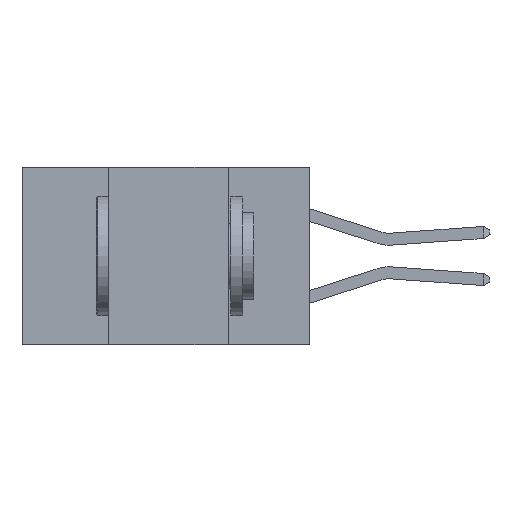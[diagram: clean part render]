
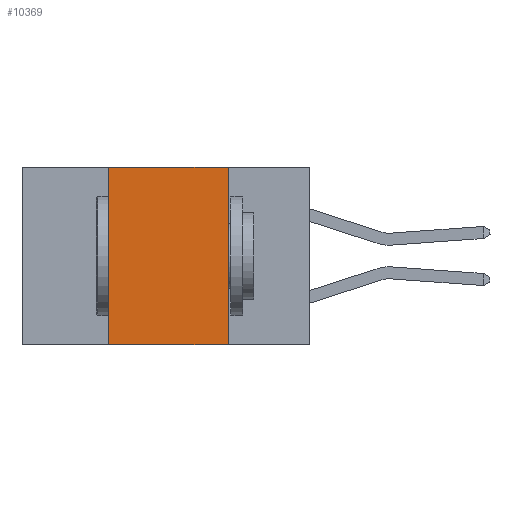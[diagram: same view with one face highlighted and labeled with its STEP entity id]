
A CAD part, left-side view. The second image highlights one B-rep face of the part: STEP entity #10369.
In plain terms, the highlighted planar face has unit normal (-1, 0, 0).
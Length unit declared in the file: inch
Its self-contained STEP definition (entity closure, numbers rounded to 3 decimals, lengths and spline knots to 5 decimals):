
#608 = DIRECTION ( 'NONE',  ( 0., -1., 0. ) ) ;
#1978 = VECTOR ( 'NONE', #22220, 39.37008 ) ;
#2486 = EDGE_CURVE ( 'NONE', #22380, #10706, #23877, .T. ) ;
#3511 = CARTESIAN_POINT ( 'NONE',  ( 0., 0.17, -0.37 ) ) ;
#4095 = CARTESIAN_POINT ( 'NONE',  ( 0., 0.42, -0.37 ) ) ;
#6187 = ORIENTED_EDGE ( 'NONE', *, *, #8507, .T. ) ;
#6933 = AXIS2_PLACEMENT_3D ( 'NONE', #25774, #12176, #10181 ) ;
#7000 = CARTESIAN_POINT ( 'NONE',  ( 0., 0.17, 0. ) ) ;
#7050 = ORIENTED_EDGE ( 'NONE', *, *, #11353, .F. ) ;
#7614 = DIRECTION ( 'NONE',  ( 0., 0., -1. ) ) ;
#8507 = EDGE_CURVE ( 'NONE', #22380, #21673, #9624, .T. ) ;
#9624 = LINE ( 'NONE', #26332, #1978 ) ;
#10181 = DIRECTION ( 'NONE',  ( 0., 0., -1. ) ) ;
#10369 = ADVANCED_FACE ( 'NONE', ( #14730 ), #17142, .F. ) ;
#10443 = DIRECTION ( 'NONE',  ( 0., 0., 1. ) ) ;
#10706 = VERTEX_POINT ( 'NONE', #25271 ) ;
#11353 = EDGE_CURVE ( 'NONE', #10706, #20570, #24352, .T. ) ;
#11477 = CARTESIAN_POINT ( 'NONE',  ( 0., 0.6, 0. ) ) ;
#12176 = DIRECTION ( 'NONE',  ( 1., 0., 0. ) ) ;
#13243 = VECTOR ( 'NONE', #7614, 39.37008 ) ;
#14121 = LINE ( 'NONE', #3511, #13243 ) ;
#14372 = CARTESIAN_POINT ( 'NONE',  ( 0., 0.17, -0.37 ) ) ;
#14730 = FACE_OUTER_BOUND ( 'NONE', #25822, .T. ) ;
#16004 = VECTOR ( 'NONE', #608, 39.37008 ) ;
#17142 = PLANE ( 'NONE',  #6933 ) ;
#17841 = ORIENTED_EDGE ( 'NONE', *, *, #26201, .F. ) ;
#18448 = VECTOR ( 'NONE', #10443, 39.37008 ) ;
#20570 = VERTEX_POINT ( 'NONE', #7000 ) ;
#21673 = VERTEX_POINT ( 'NONE', #14372 ) ;
#22220 = DIRECTION ( 'NONE',  ( 0., -1., 0. ) ) ;
#22380 = VERTEX_POINT ( 'NONE', #26205 ) ;
#23877 = LINE ( 'NONE', #4095, #18448 ) ;
#24352 = LINE ( 'NONE', #11477, #16004 ) ;
#25271 = CARTESIAN_POINT ( 'NONE',  ( 0., 0.42, 0. ) ) ;
#25289 = ORIENTED_EDGE ( 'NONE', *, *, #2486, .F. ) ;
#25774 = CARTESIAN_POINT ( 'NONE',  ( 0., 0.6, 0. ) ) ;
#25822 = EDGE_LOOP ( 'NONE', ( #17841, #7050, #25289, #6187 ) ) ;
#26201 = EDGE_CURVE ( 'NONE', #20570, #21673, #14121, .T. ) ;
#26205 = CARTESIAN_POINT ( 'NONE',  ( 0., 0.42, -0.37 ) ) ;
#26332 = CARTESIAN_POINT ( 'NONE',  ( 0., 0.6, -0.37 ) ) ;
